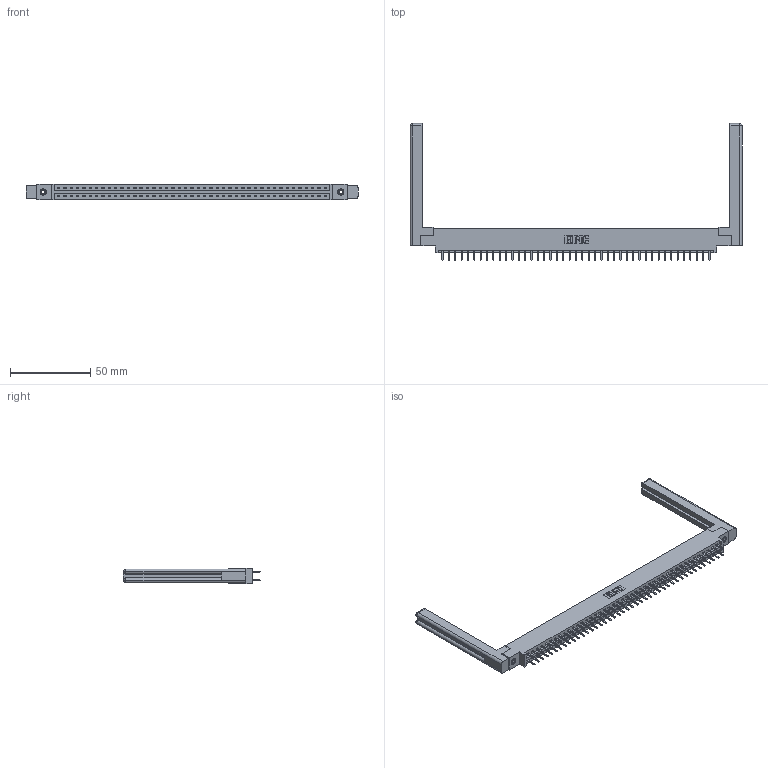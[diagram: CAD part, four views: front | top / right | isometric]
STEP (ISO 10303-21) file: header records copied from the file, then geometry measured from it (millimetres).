
FILE_DESCRIPTION (( 'STEP AP203' ), '1' );
FILE_NAME ('387-086-520-858.STEP', '2019-10-23T02:49:57', ( '' ), ( '' ), 'SwSTEP 2.0', 'SolidWorks 2016', '' );
FILE_SCHEMA (( 'CONFIG_CONTROL_DESIGN' ));
Length unit declared in the file: inch
Products named in the file (5): 307-220-058; 337 Part_0.170 Offset - 0.156 Dia-TI; 345-292-001_345-293-120; 387-086-520-858; 345-250-001_345-250-001-102
Assembly tree (91 placements, depth 2):
  387-086-520-858
    337 Part_0.170 Offset - 0.156 Dia-TI
    345-292-001_345-293-120  x86
    345-250-001_345-250-001-102  x2
    307-220-058  x2
Bounding box: 207.01 x 85.43 x 9.4 mm (x, y, z)
Volume: 28816.7 mm3; surface area: 29559.4 mm2
Topology: 91 solids, 91 shells, 5248 faces, 15211 edges, 9898 vertices
Faces by surface type: plane 3598, cylinder 1626, cone 12, torus 12
Entity records: 36090 total; most frequent: CARTESIAN_POINT 6101, ORIENTED_EDGE 5964, DIRECTION 5190, EDGE_CURVE 2982, LINE 2802, VECTOR 2802, VERTEX_POINT 1978, AXIS2_PLACEMENT_3D 1194
